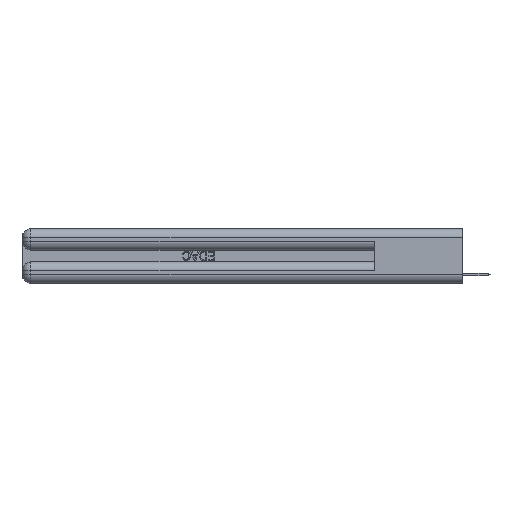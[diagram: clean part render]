
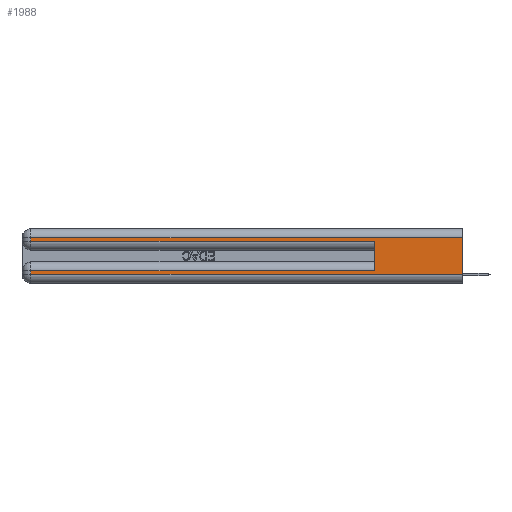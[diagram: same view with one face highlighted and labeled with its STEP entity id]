
A CAD part, left-side view. The second image highlights one B-rep face of the part: STEP entity #1988.
In plain terms, the highlighted planar face has unit normal (-1, 0, 0).
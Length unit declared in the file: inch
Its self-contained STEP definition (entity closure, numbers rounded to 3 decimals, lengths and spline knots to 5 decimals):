
#1237 = LINE ( 'NONE', #23114, #22848 ) ;
#1275 = VECTOR ( 'NONE', #15509, 39.37008 ) ;
#1384 = LINE ( 'NONE', #20730, #1275 ) ;
#1836 = DIRECTION ( 'NONE',  ( 1., 0., 0. ) ) ;
#1988 = ADVANCED_FACE ( 'NONE', ( #16122 ), #4386, .F. ) ;
#2269 = ORIENTED_EDGE ( 'NONE', *, *, #26731, .T. ) ;
#2551 = ORIENTED_EDGE ( 'NONE', *, *, #6612, .T. ) ;
#2675 = DIRECTION ( 'NONE',  ( 0., 0., 1. ) ) ;
#2741 = CARTESIAN_POINT ( 'NONE',  ( 0., 0., 0.31 ) ) ;
#2994 = CARTESIAN_POINT ( 'NONE',  ( 0., 0.6, 0.145 ) ) ;
#4133 = CARTESIAN_POINT ( 'NONE',  ( 0., 2.94, 0.285 ) ) ;
#4335 = EDGE_CURVE ( 'NONE', #12597, #19499, #21862, .T. ) ;
#4386 = PLANE ( 'NONE',  #20470 ) ;
#4696 = EDGE_CURVE ( 'NONE', #23413, #28930, #30849, .T. ) ;
#4705 = DIRECTION ( 'NONE',  ( 0., 0., -1. ) ) ;
#4752 = VERTEX_POINT ( 'NONE', #4778 ) ;
#4778 = CARTESIAN_POINT ( 'NONE',  ( 0., 0., 0.06 ) ) ;
#5812 = VECTOR ( 'NONE', #30493, 39.37008 ) ;
#6311 = DIRECTION ( 'NONE',  ( 0., 1., 0. ) ) ;
#6549 = CARTESIAN_POINT ( 'NONE',  ( 0., 2.94, 0.31 ) ) ;
#6612 = EDGE_CURVE ( 'NONE', #15766, #19499, #1384, .T. ) ;
#6861 = VERTEX_POINT ( 'NONE', #21823 ) ;
#8612 = EDGE_LOOP ( 'NONE', ( #12369, #12030, #30743, #2551, #12654, #29729, #25050, #2269 ) ) ;
#10868 = CARTESIAN_POINT ( 'NONE',  ( 0., 0., 0.06 ) ) ;
#11361 = CARTESIAN_POINT ( 'NONE',  ( 0., 0.6, 0.285 ) ) ;
#11698 = LINE ( 'NONE', #13910, #26718 ) ;
#11986 = EDGE_CURVE ( 'NONE', #28639, #6861, #1237, .T. ) ;
#12030 = ORIENTED_EDGE ( 'NONE', *, *, #4696, .T. ) ;
#12369 = ORIENTED_EDGE ( 'NONE', *, *, #13329, .F. ) ;
#12554 = CARTESIAN_POINT ( 'NONE',  ( 0., 0.6, 0.085 ) ) ;
#12597 = VERTEX_POINT ( 'NONE', #12554 ) ;
#12654 = ORIENTED_EDGE ( 'NONE', *, *, #4335, .F. ) ;
#12687 = LINE ( 'NONE', #22329, #20060 ) ;
#13329 = EDGE_CURVE ( 'NONE', #23413, #4752, #11698, .T. ) ;
#13910 = CARTESIAN_POINT ( 'NONE',  ( 0., 0., 0.37 ) ) ;
#13945 = LINE ( 'NONE', #23596, #24881 ) ;
#15509 = DIRECTION ( 'NONE',  ( 0., -1., 0. ) ) ;
#15766 = VERTEX_POINT ( 'NONE', #4133 ) ;
#16122 = FACE_OUTER_BOUND ( 'NONE', #8612, .T. ) ;
#18510 = CARTESIAN_POINT ( 'NONE',  ( 0., 0., 0.31 ) ) ;
#18782 = LINE ( 'NONE', #10868, #5812 ) ;
#19249 = CARTESIAN_POINT ( 'NONE',  ( 0., 2.94, 0.085 ) ) ;
#19499 = VERTEX_POINT ( 'NONE', #11361 ) ;
#20060 = VECTOR ( 'NONE', #23578, 39.37008 ) ;
#20470 = AXIS2_PLACEMENT_3D ( 'NONE', #23555, #1836, #25784 ) ;
#20730 = CARTESIAN_POINT ( 'NONE',  ( 0., 0., 0.285 ) ) ;
#21101 = EDGE_CURVE ( 'NONE', #12597, #28639, #13945, .T. ) ;
#21823 = CARTESIAN_POINT ( 'NONE',  ( 0., 2.94, 0.06 ) ) ;
#21862 = LINE ( 'NONE', #2994, #25075 ) ;
#22329 = CARTESIAN_POINT ( 'NONE',  ( 0., 2.94, 0.37 ) ) ;
#22848 = VECTOR ( 'NONE', #25808, 39.37008 ) ;
#23114 = CARTESIAN_POINT ( 'NONE',  ( 0., 2.94, 0.37 ) ) ;
#23413 = VERTEX_POINT ( 'NONE', #2741 ) ;
#23555 = CARTESIAN_POINT ( 'NONE',  ( 0., 0., 0.37 ) ) ;
#23578 = DIRECTION ( 'NONE',  ( 0., 0., -1. ) ) ;
#23596 = CARTESIAN_POINT ( 'NONE',  ( 0., 0., 0.085 ) ) ;
#24881 = VECTOR ( 'NONE', #31026, 39.37008 ) ;
#25050 = ORIENTED_EDGE ( 'NONE', *, *, #11986, .T. ) ;
#25075 = VECTOR ( 'NONE', #2675, 39.37008 ) ;
#25784 = DIRECTION ( 'NONE',  ( 0., 0., -1. ) ) ;
#25808 = DIRECTION ( 'NONE',  ( 0., 0., -1. ) ) ;
#26718 = VECTOR ( 'NONE', #4705, 39.37008 ) ;
#26731 = EDGE_CURVE ( 'NONE', #6861, #4752, #18782, .T. ) ;
#28639 = VERTEX_POINT ( 'NONE', #19249 ) ;
#28930 = VERTEX_POINT ( 'NONE', #6549 ) ;
#29706 = EDGE_CURVE ( 'NONE', #28930, #15766, #12687, .T. ) ;
#29729 = ORIENTED_EDGE ( 'NONE', *, *, #21101, .T. ) ;
#30306 = VECTOR ( 'NONE', #6311, 39.37008 ) ;
#30493 = DIRECTION ( 'NONE',  ( 0., -1., 0. ) ) ;
#30743 = ORIENTED_EDGE ( 'NONE', *, *, #29706, .T. ) ;
#30849 = LINE ( 'NONE', #18510, #30306 ) ;
#31026 = DIRECTION ( 'NONE',  ( 0., 1., 0. ) ) ;
